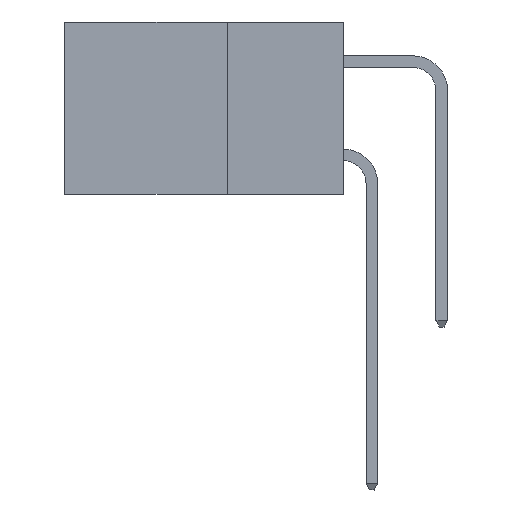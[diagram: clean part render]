
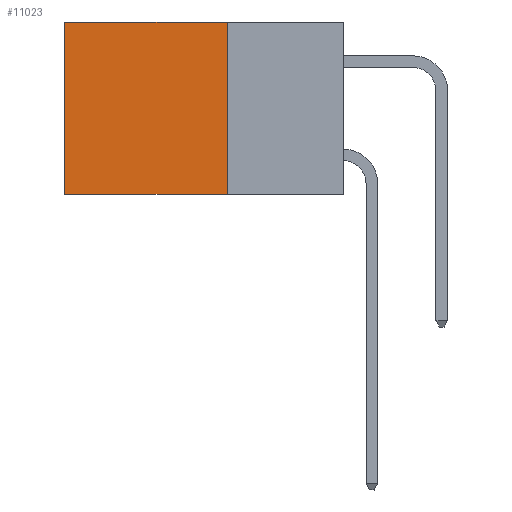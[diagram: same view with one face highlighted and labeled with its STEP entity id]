
A CAD part, left-side view. The second image highlights one B-rep face of the part: STEP entity #11023.
In plain terms, the highlighted planar face has unit normal (-1, 0, 0).
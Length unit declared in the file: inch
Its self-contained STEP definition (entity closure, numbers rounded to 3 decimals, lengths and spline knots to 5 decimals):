
#246 = EDGE_CURVE ( 'NONE', #18585, #14795, #9148, .T. ) ;
#620 = VECTOR ( 'NONE', #2829, 39.37008 ) ;
#781 = DIRECTION ( 'NONE',  ( 0., 0., -1. ) ) ;
#1876 = DIRECTION ( 'NONE',  ( 0., 1., 0. ) ) ;
#1928 = CARTESIAN_POINT ( 'NONE',  ( 0.298, 0.25, 0. ) ) ;
#2829 = DIRECTION ( 'NONE',  ( 0., 1., 0. ) ) ;
#2940 = CARTESIAN_POINT ( 'NONE',  ( 0.298, 0.25, -0.37 ) ) ;
#3656 = ORIENTED_EDGE ( 'NONE', *, *, #7623, .F. ) ;
#4755 = CARTESIAN_POINT ( 'NONE',  ( 0.298, 0.25, 0. ) ) ;
#5853 = LINE ( 'NONE', #5935, #13729 ) ;
#5875 = DIRECTION ( 'NONE',  ( 0., 0., -1. ) ) ;
#5935 = CARTESIAN_POINT ( 'NONE',  ( 0.298, 0.25, 0. ) ) ;
#6227 = CARTESIAN_POINT ( 'NONE',  ( 0.298, 0.6, -0.37 ) ) ;
#7099 = EDGE_CURVE ( 'NONE', #12722, #12929, #12540, .T. ) ;
#7198 = PLANE ( 'NONE',  #17286 ) ;
#7353 = VECTOR ( 'NONE', #1876, 39.37008 ) ;
#7623 = EDGE_CURVE ( 'NONE', #12722, #18585, #5853, .T. ) ;
#7940 = VECTOR ( 'NONE', #9839, 39.37008 ) ;
#8497 = CARTESIAN_POINT ( 'NONE',  ( 0.298, 0.6, 0. ) ) ;
#9148 = LINE ( 'NONE', #13340, #620 ) ;
#9743 = CARTESIAN_POINT ( 'NONE',  ( 0.298, 0.6, 0. ) ) ;
#9839 = DIRECTION ( 'NONE',  ( 0., 0., -1. ) ) ;
#10238 = EDGE_CURVE ( 'NONE', #12929, #14795, #16210, .T. ) ;
#10335 = DIRECTION ( 'NONE',  ( 1., 0., 0. ) ) ;
#10664 = ORIENTED_EDGE ( 'NONE', *, *, #10238, .T. ) ;
#10876 = ORIENTED_EDGE ( 'NONE', *, *, #7099, .T. ) ;
#11023 = ADVANCED_FACE ( 'NONE', ( #13588 ), #7198, .F. ) ;
#11714 = ORIENTED_EDGE ( 'NONE', *, *, #246, .F. ) ;
#12540 = LINE ( 'NONE', #1928, #7353 ) ;
#12722 = VERTEX_POINT ( 'NONE', #4755 ) ;
#12929 = VERTEX_POINT ( 'NONE', #8497 ) ;
#13340 = CARTESIAN_POINT ( 'NONE',  ( 0.298, 0.25, -0.37 ) ) ;
#13588 = FACE_OUTER_BOUND ( 'NONE', #19537, .T. ) ;
#13729 = VECTOR ( 'NONE', #5875, 39.37008 ) ;
#14795 = VERTEX_POINT ( 'NONE', #6227 ) ;
#16210 = LINE ( 'NONE', #9743, #7940 ) ;
#17286 = AXIS2_PLACEMENT_3D ( 'NONE', #19450, #10335, #781 ) ;
#18585 = VERTEX_POINT ( 'NONE', #2940 ) ;
#19450 = CARTESIAN_POINT ( 'NONE',  ( 0.298, 0.25, 0. ) ) ;
#19537 = EDGE_LOOP ( 'NONE', ( #10664, #11714, #3656, #10876 ) ) ;
